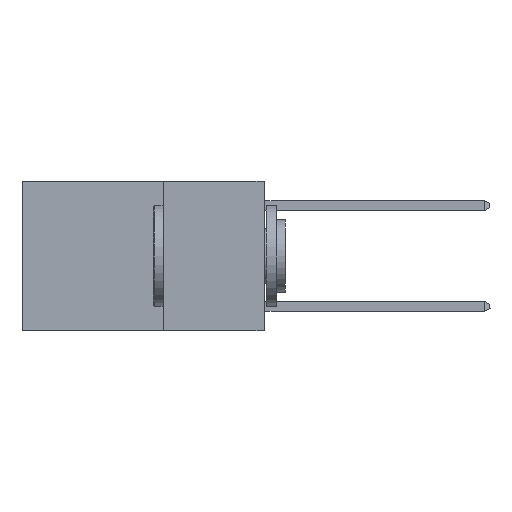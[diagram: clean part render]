
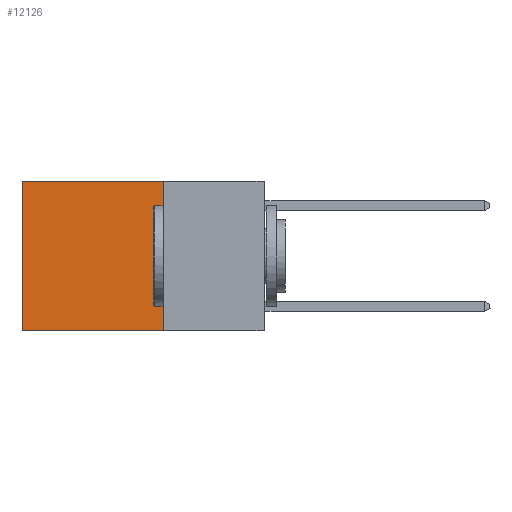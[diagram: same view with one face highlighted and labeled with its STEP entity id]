
A CAD part, left-side view. The second image highlights one B-rep face of the part: STEP entity #12126.
In plain terms, the highlighted planar face has unit normal (-1, 0, 0).
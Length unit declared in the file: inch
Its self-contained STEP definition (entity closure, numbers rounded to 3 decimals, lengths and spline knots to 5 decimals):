
#623 = VERTEX_POINT ( 'NONE', #17707 ) ;
#946 = ORIENTED_EDGE ( 'NONE', *, *, #11253, .F. ) ;
#1454 = CARTESIAN_POINT ( 'NONE',  ( 0.2625, 0.25, 0. ) ) ;
#1771 = LINE ( 'NONE', #4310, #8898 ) ;
#3168 = VERTEX_POINT ( 'NONE', #4049 ) ;
#3694 = ORIENTED_EDGE ( 'NONE', *, *, #14888, .T. ) ;
#4049 = CARTESIAN_POINT ( 'NONE',  ( 0.2625, 0.25, -0.37 ) ) ;
#4264 = CARTESIAN_POINT ( 'NONE',  ( 0.2625, 0.25, 0. ) ) ;
#4310 = CARTESIAN_POINT ( 'NONE',  ( 0.2625, 0.25, -0.37 ) ) ;
#5575 = VERTEX_POINT ( 'NONE', #15065 ) ;
#5777 = DIRECTION ( 'NONE',  ( 0., 1., 0. ) ) ;
#5920 = DIRECTION ( 'NONE',  ( 0., 1., 0. ) ) ;
#6037 = CARTESIAN_POINT ( 'NONE',  ( 0.2625, 0.6, 0. ) ) ;
#6319 = LINE ( 'NONE', #17846, #15768 ) ;
#8199 = LINE ( 'NONE', #9628, #13355 ) ;
#8527 = FACE_OUTER_BOUND ( 'NONE', #11796, .T. ) ;
#8898 = VECTOR ( 'NONE', #5920, 39.37008 ) ;
#9206 = VERTEX_POINT ( 'NONE', #6037 ) ;
#9243 = AXIS2_PLACEMENT_3D ( 'NONE', #4264, #11460, #10040 ) ;
#9628 = CARTESIAN_POINT ( 'NONE',  ( 0.2625, 0.25, 0. ) ) ;
#10040 = DIRECTION ( 'NONE',  ( 0., 0., -1. ) ) ;
#11253 = EDGE_CURVE ( 'NONE', #3168, #623, #1771, .T. ) ;
#11460 = DIRECTION ( 'NONE',  ( 1., 0., 0. ) ) ;
#11796 = EDGE_LOOP ( 'NONE', ( #16125, #946, #14125, #3694 ) ) ;
#12126 = ADVANCED_FACE ( 'NONE', ( #8527 ), #15623, .F. ) ;
#13355 = VECTOR ( 'NONE', #15576, 39.37008 ) ;
#14125 = ORIENTED_EDGE ( 'NONE', *, *, #15903, .F. ) ;
#14404 = LINE ( 'NONE', #1454, #18313 ) ;
#14888 = EDGE_CURVE ( 'NONE', #5575, #9206, #14404, .T. ) ;
#15065 = CARTESIAN_POINT ( 'NONE',  ( 0.2625, 0.25, 0. ) ) ;
#15576 = DIRECTION ( 'NONE',  ( 0., 0., -1. ) ) ;
#15623 = PLANE ( 'NONE',  #9243 ) ;
#15768 = VECTOR ( 'NONE', #16259, 39.37008 ) ;
#15809 = EDGE_CURVE ( 'NONE', #9206, #623, #6319, .T. ) ;
#15903 = EDGE_CURVE ( 'NONE', #5575, #3168, #8199, .T. ) ;
#16125 = ORIENTED_EDGE ( 'NONE', *, *, #15809, .T. ) ;
#16259 = DIRECTION ( 'NONE',  ( 0., 0., -1. ) ) ;
#17707 = CARTESIAN_POINT ( 'NONE',  ( 0.2625, 0.6, -0.37 ) ) ;
#17846 = CARTESIAN_POINT ( 'NONE',  ( 0.2625, 0.6, 0. ) ) ;
#18313 = VECTOR ( 'NONE', #5777, 39.37008 ) ;
